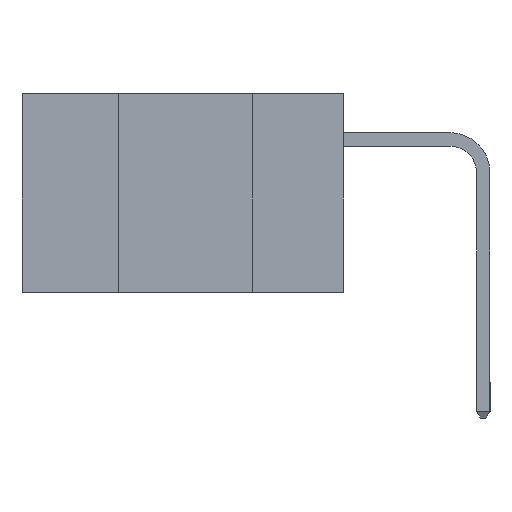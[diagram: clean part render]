
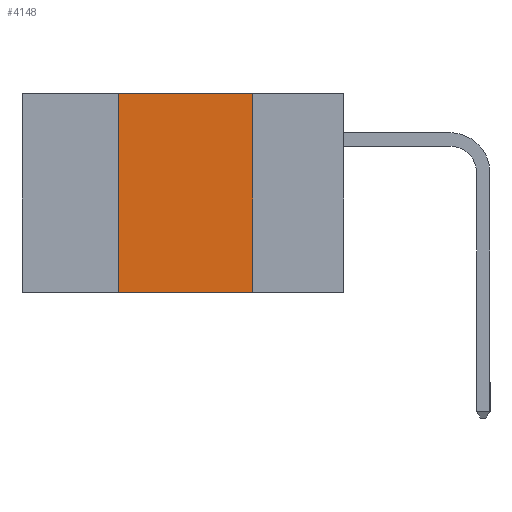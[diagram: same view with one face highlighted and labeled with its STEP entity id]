
A CAD part, left-side view. The second image highlights one B-rep face of the part: STEP entity #4148.
In plain terms, the highlighted planar face has unit normal (-1, 0, 0).
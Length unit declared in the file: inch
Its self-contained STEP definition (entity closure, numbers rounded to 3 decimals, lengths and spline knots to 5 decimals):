
#87 = DIRECTION ( 'NONE',  ( 0., 0., -1. ) ) ;
#373 = DIRECTION ( 'NONE',  ( 0., -1., 0. ) ) ;
#826 = EDGE_LOOP ( 'NONE', ( #1127, #1140, #7295, #7100 ) ) ;
#1127 = ORIENTED_EDGE ( 'NONE', *, *, #3865, .F. ) ;
#1140 = ORIENTED_EDGE ( 'NONE', *, *, #3015, .F. ) ;
#1349 = CARTESIAN_POINT ( 'NONE',  ( 0., 0.6, 0. ) ) ;
#2291 = LINE ( 'NONE', #8992, #10430 ) ;
#2930 = VECTOR ( 'NONE', #9751, 39.37008 ) ;
#3015 = EDGE_CURVE ( 'NONE', #8061, #12416, #10257, .T. ) ;
#3489 = CARTESIAN_POINT ( 'NONE',  ( 0., 0.17, 0. ) ) ;
#3865 = EDGE_CURVE ( 'NONE', #12416, #7866, #2291, .T. ) ;
#4097 = CARTESIAN_POINT ( 'NONE',  ( 0., 0.42, 0. ) ) ;
#4148 = ADVANCED_FACE ( 'NONE', ( #5842 ), #10847, .F. ) ;
#4286 = DIRECTION ( 'NONE',  ( 1., 0., 0. ) ) ;
#4364 = CARTESIAN_POINT ( 'NONE',  ( 0., 0.17, -0.37 ) ) ;
#4409 = CARTESIAN_POINT ( 'NONE',  ( 0., 0.6, 0. ) ) ;
#4630 = LINE ( 'NONE', #6578, #2930 ) ;
#5842 = FACE_OUTER_BOUND ( 'NONE', #826, .T. ) ;
#6578 = CARTESIAN_POINT ( 'NONE',  ( 0., 0.6, -0.37 ) ) ;
#7034 = VERTEX_POINT ( 'NONE', #9066 ) ;
#7100 = ORIENTED_EDGE ( 'NONE', *, *, #9539, .T. ) ;
#7295 = ORIENTED_EDGE ( 'NONE', *, *, #9521, .F. ) ;
#7866 = VERTEX_POINT ( 'NONE', #4364 ) ;
#8061 = VERTEX_POINT ( 'NONE', #4097 ) ;
#8992 = CARTESIAN_POINT ( 'NONE',  ( 0., 0.17, -0.37 ) ) ;
#9066 = CARTESIAN_POINT ( 'NONE',  ( 0., 0.42, -0.37 ) ) ;
#9521 = EDGE_CURVE ( 'NONE', #7034, #8061, #10678, .T. ) ;
#9537 = AXIS2_PLACEMENT_3D ( 'NONE', #4409, #4286, #10259 ) ;
#9539 = EDGE_CURVE ( 'NONE', #7034, #7866, #4630, .T. ) ;
#9751 = DIRECTION ( 'NONE',  ( 0., -1., 0. ) ) ;
#10257 = LINE ( 'NONE', #1349, #12287 ) ;
#10259 = DIRECTION ( 'NONE',  ( 0., 0., -1. ) ) ;
#10430 = VECTOR ( 'NONE', #87, 39.37008 ) ;
#10608 = DIRECTION ( 'NONE',  ( 0., 0., 1. ) ) ;
#10678 = LINE ( 'NONE', #12857, #12750 ) ;
#10847 = PLANE ( 'NONE',  #9537 ) ;
#12287 = VECTOR ( 'NONE', #373, 39.37008 ) ;
#12416 = VERTEX_POINT ( 'NONE', #3489 ) ;
#12750 = VECTOR ( 'NONE', #10608, 39.37008 ) ;
#12857 = CARTESIAN_POINT ( 'NONE',  ( 0., 0.42, -0.37 ) ) ;
